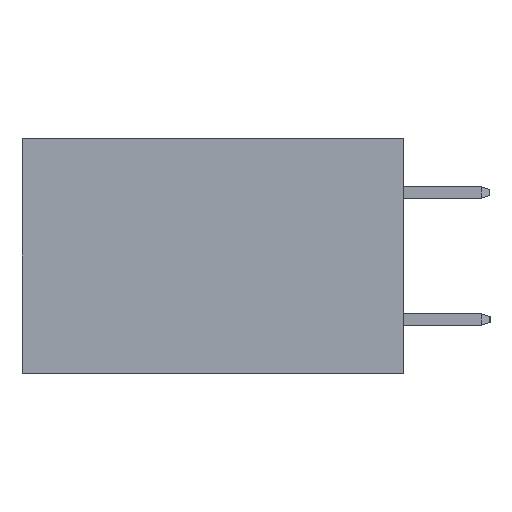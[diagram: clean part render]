
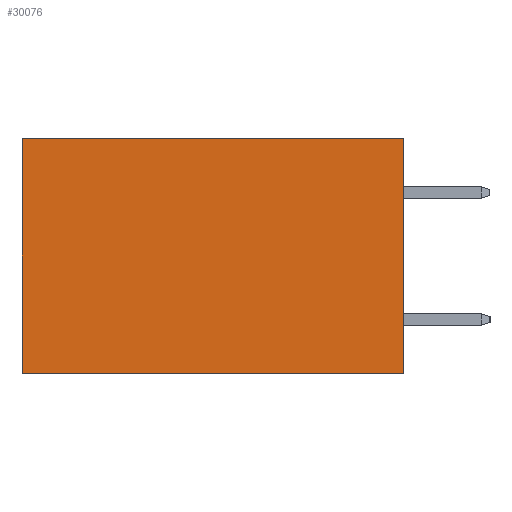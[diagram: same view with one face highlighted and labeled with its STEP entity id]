
A CAD part, left-side view. The second image highlights one B-rep face of the part: STEP entity #30076.
In plain terms, the highlighted planar face has unit normal (-1, 0, 0).
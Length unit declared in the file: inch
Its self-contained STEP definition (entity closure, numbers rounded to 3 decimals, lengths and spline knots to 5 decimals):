
#883 = EDGE_CURVE ( 'NONE', #24495, #6354, #30097, .T. ) ;
#926 = CARTESIAN_POINT ( 'NONE',  ( 0.2875, 0., -0.37 ) ) ;
#1528 = ORIENTED_EDGE ( 'NONE', *, *, #20562, .F. ) ;
#1928 = DIRECTION ( 'NONE',  ( 0., 1., 0. ) ) ;
#2646 = VECTOR ( 'NONE', #24822, 39.37008 ) ;
#2728 = ORIENTED_EDGE ( 'NONE', *, *, #33215, .T. ) ;
#3343 = VECTOR ( 'NONE', #23942, 39.37008 ) ;
#3607 = LINE ( 'NONE', #22268, #2646 ) ;
#4728 = DIRECTION ( 'NONE',  ( 1., 0., 0. ) ) ;
#5299 = CARTESIAN_POINT ( 'NONE',  ( 0.2875, 0.6, 0. ) ) ;
#6354 = VERTEX_POINT ( 'NONE', #13275 ) ;
#7617 = LINE ( 'NONE', #24482, #3343 ) ;
#11916 = ORIENTED_EDGE ( 'NONE', *, *, #883, .T. ) ;
#12112 = CARTESIAN_POINT ( 'NONE',  ( 0.2875, 0.6, 0. ) ) ;
#13275 = CARTESIAN_POINT ( 'NONE',  ( 0.2875, 0.6, -0.37 ) ) ;
#16324 = DIRECTION ( 'NONE',  ( 0., 0., -1. ) ) ;
#17848 = VECTOR ( 'NONE', #1928, 39.37008 ) ;
#18603 = CARTESIAN_POINT ( 'NONE',  ( 0.2875, 0., 0. ) ) ;
#19128 = ORIENTED_EDGE ( 'NONE', *, *, #24275, .F. ) ;
#20562 = EDGE_CURVE ( 'NONE', #22913, #6354, #3607, .T. ) ;
#21578 = DIRECTION ( 'NONE',  ( 0., 0., -1. ) ) ;
#22268 = CARTESIAN_POINT ( 'NONE',  ( 0.2875, 0., -0.37 ) ) ;
#22913 = VERTEX_POINT ( 'NONE', #926 ) ;
#23593 = VERTEX_POINT ( 'NONE', #25829 ) ;
#23874 = LINE ( 'NONE', #18603, #17848 ) ;
#23942 = DIRECTION ( 'NONE',  ( 0., 0., -1. ) ) ;
#24275 = EDGE_CURVE ( 'NONE', #23593, #22913, #7617, .T. ) ;
#24482 = CARTESIAN_POINT ( 'NONE',  ( 0.2875, 0., 0. ) ) ;
#24495 = VERTEX_POINT ( 'NONE', #12112 ) ;
#24822 = DIRECTION ( 'NONE',  ( 0., 1., 0. ) ) ;
#25829 = CARTESIAN_POINT ( 'NONE',  ( 0.2875, 0., 0. ) ) ;
#26981 = PLANE ( 'NONE',  #27299 ) ;
#27299 = AXIS2_PLACEMENT_3D ( 'NONE', #29696, #4728, #21578 ) ;
#28368 = VECTOR ( 'NONE', #16324, 39.37008 ) ;
#28483 = EDGE_LOOP ( 'NONE', ( #11916, #1528, #19128, #2728 ) ) ;
#29696 = CARTESIAN_POINT ( 'NONE',  ( 0.2875, 0., 0. ) ) ;
#30076 = ADVANCED_FACE ( 'NONE', ( #34982 ), #26981, .F. ) ;
#30097 = LINE ( 'NONE', #5299, #28368 ) ;
#33215 = EDGE_CURVE ( 'NONE', #23593, #24495, #23874, .T. ) ;
#34982 = FACE_OUTER_BOUND ( 'NONE', #28483, .T. ) ;
